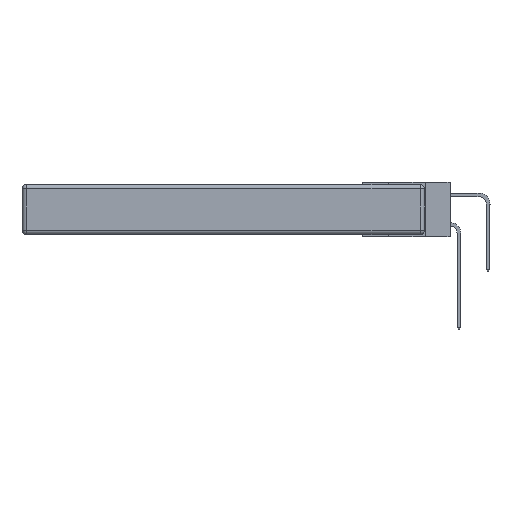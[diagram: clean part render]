
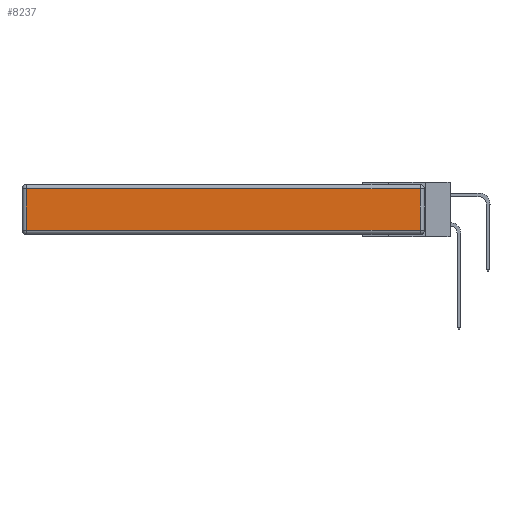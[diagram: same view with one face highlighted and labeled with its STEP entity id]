
A CAD part, left-side view. The second image highlights one B-rep face of the part: STEP entity #8237.
In plain terms, the highlighted planar face has unit normal (-1, 0, 0).
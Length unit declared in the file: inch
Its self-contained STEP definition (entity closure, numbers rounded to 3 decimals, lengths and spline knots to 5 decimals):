
#887 = EDGE_CURVE ( 'NONE', #15201, #1430, #12519, .T. ) ;
#1221 = CARTESIAN_POINT ( 'NONE',  ( 0., 2.75, -0.03 ) ) ;
#1356 = EDGE_CURVE ( 'NONE', #4631, #6161, #16834, .T. ) ;
#1401 = CARTESIAN_POINT ( 'NONE',  ( 0., 0.03, -0.343 ) ) ;
#1430 = VERTEX_POINT ( 'NONE', #7035 ) ;
#1573 = LINE ( 'NONE', #1401, #7786 ) ;
#1785 = ORIENTED_EDGE ( 'NONE', *, *, #19280, .T. ) ;
#2429 = ORIENTED_EDGE ( 'NONE', *, *, #10677, .T. ) ;
#2834 = CARTESIAN_POINT ( 'NONE',  ( 0., 0.03, -0.03 ) ) ;
#4631 = VERTEX_POINT ( 'NONE', #4881 ) ;
#4881 = CARTESIAN_POINT ( 'NONE',  ( 0., 2.72, -0.313 ) ) ;
#4974 = DIRECTION ( 'NONE',  ( -1., 0., 0. ) ) ;
#5565 = CARTESIAN_POINT ( 'NONE',  ( 0., 0., -0.313 ) ) ;
#5575 = VECTOR ( 'NONE', #6963, 39.37008 ) ;
#6161 = VERTEX_POINT ( 'NONE', #16856 ) ;
#6963 = DIRECTION ( 'NONE',  ( 0., -1., 0. ) ) ;
#7035 = CARTESIAN_POINT ( 'NONE',  ( 0., 2.72, -0.03 ) ) ;
#7786 = VECTOR ( 'NONE', #13437, 39.37008 ) ;
#8171 = DIRECTION ( 'NONE',  ( 0., 0., -1. ) ) ;
#8230 = CARTESIAN_POINT ( 'NONE',  ( 0., 0., -0.343 ) ) ;
#8237 = ADVANCED_FACE ( 'NONE', ( #11542 ), #9491, .T. ) ;
#9491 = PLANE ( 'NONE',  #17543 ) ;
#10677 = EDGE_CURVE ( 'NONE', #1430, #4631, #11360, .T. ) ;
#11360 = LINE ( 'NONE', #15918, #12347 ) ;
#11542 = FACE_OUTER_BOUND ( 'NONE', #13535, .T. ) ;
#12296 = VECTOR ( 'NONE', #17840, 39.37008 ) ;
#12347 = VECTOR ( 'NONE', #8171, 39.37008 ) ;
#12519 = LINE ( 'NONE', #1221, #12296 ) ;
#13437 = DIRECTION ( 'NONE',  ( 0., 0., 1. ) ) ;
#13535 = EDGE_LOOP ( 'NONE', ( #17004, #1785, #19285, #2429 ) ) ;
#15201 = VERTEX_POINT ( 'NONE', #2834 ) ;
#15658 = DIRECTION ( 'NONE',  ( 0., 0., 1. ) ) ;
#15918 = CARTESIAN_POINT ( 'NONE',  ( 0., 2.72, -0.343 ) ) ;
#16834 = LINE ( 'NONE', #5565, #5575 ) ;
#16856 = CARTESIAN_POINT ( 'NONE',  ( 0., 0.03, -0.313 ) ) ;
#17004 = ORIENTED_EDGE ( 'NONE', *, *, #1356, .T. ) ;
#17543 = AXIS2_PLACEMENT_3D ( 'NONE', #8230, #4974, #15658 ) ;
#17840 = DIRECTION ( 'NONE',  ( 0., 1., 0. ) ) ;
#19280 = EDGE_CURVE ( 'NONE', #6161, #15201, #1573, .T. ) ;
#19285 = ORIENTED_EDGE ( 'NONE', *, *, #887, .T. ) ;
